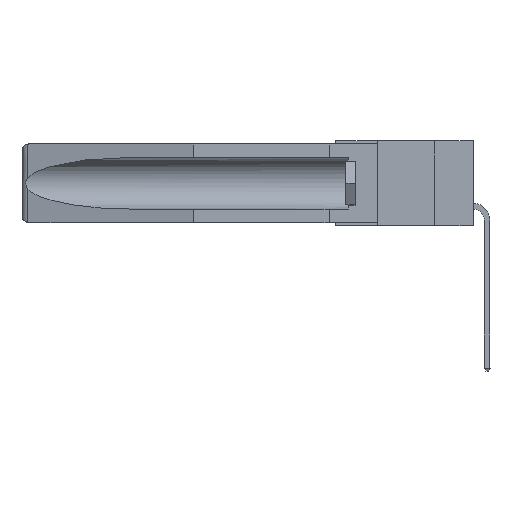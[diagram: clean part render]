
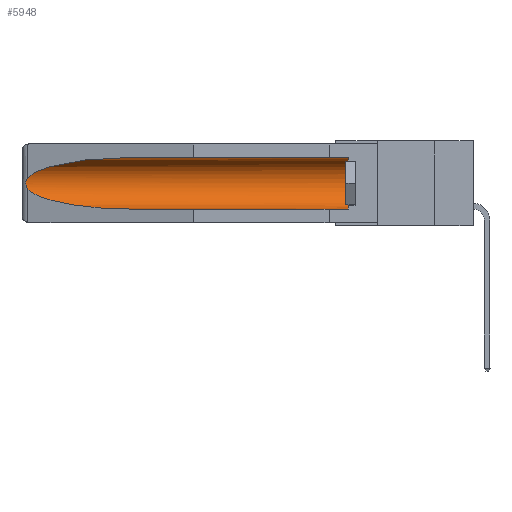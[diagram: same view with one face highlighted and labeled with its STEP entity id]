
A CAD part, left-side view. The second image highlights one B-rep face of the part: STEP entity #5948.
In plain terms, the highlighted cylindrical face has radius 2.857 mm (diameter 5.715 mm), a partial arc.
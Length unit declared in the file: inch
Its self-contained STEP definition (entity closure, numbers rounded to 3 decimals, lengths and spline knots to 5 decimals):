
#572 = CARTESIAN_POINT ( 'NONE',  ( 0.21114, 1.30732, -0.284 ) ) ;
#575 = ORIENTED_EDGE ( 'NONE', *, *, #4611, .T. ) ;
#780 = VERTEX_POINT ( 'NONE', #11968 ) ;
#1083 = EDGE_CURVE ( 'NONE', #9374, #9616, #26352, .T. ) ;
#1348 = CARTESIAN_POINT ( 'NONE',  ( 0.2675, 1.53308, -0.16763 ) ) ;
#1921 = CARTESIAN_POINT ( 'NONE',  ( 0.21114, 1.30732, -0.059 ) ) ;
#2210 = CARTESIAN_POINT ( 'NONE',  ( 0.155, 1.07973, -0.284 ) ) ;
#2550 = EDGE_LOOP ( 'NONE', ( #8007, #18191, #14293, #14109, #11131, #575 ) ) ;
#2733 = DIRECTION ( 'NONE',  ( 0., 0., 1. ) ) ;
#3683 = LINE ( 'NONE', #10826, #23333 ) ;
#4297 =( BOUNDED_CURVE ( )  B_SPLINE_CURVE ( 3, ( #20562, #16337, #572, #22596 ),
 .UNSPECIFIED., .F., .F. ) 
 B_SPLINE_CURVE_WITH_KNOTS ( ( 4, 4 ),
 ( 0.1948, 1.5708 ),
 .UNSPECIFIED. ) 
 CURVE ( )  GEOMETRIC_REPRESENTATION_ITEM ( )  RATIONAL_B_SPLINE_CURVE ( ( 1., 0.848, 0.848, 1. ) ) 
 REPRESENTATION_ITEM ( '' )  );
#4358 = CYLINDRICAL_SURFACE ( 'NONE', #18784, 0.1125 ) ;
#4552 = DIRECTION ( 'NONE',  ( 0., 0., 1. ) ) ;
#4611 = EDGE_CURVE ( 'NONE', #9616, #21609, #3683, .T. ) ;
#4628 = CARTESIAN_POINT ( 'NONE',  ( 0.155, 1.07973, -0.059 ) ) ;
#5948 = ADVANCED_FACE ( 'NONE', ( #7500 ), #4358, .F. ) ;
#7500 = FACE_OUTER_BOUND ( 'NONE', #2550, .T. ) ;
#8007 = ORIENTED_EDGE ( 'NONE', *, *, #20783, .T. ) ;
#8088 = CARTESIAN_POINT ( 'NONE',  ( 0.26597, 1.52961, -0.15275 ) ) ;
#8586 = CARTESIAN_POINT ( 'NONE',  ( 0.155, -0.30754, -0.284 ) ) ;
#8942 = AXIS2_PLACEMENT_3D ( 'NONE', #10487, #15095, #2733 ) ;
#9217 = CARTESIAN_POINT ( 'NONE',  ( 0.26537, 1.52718, -0.14972 ) ) ;
#9374 = VERTEX_POINT ( 'NONE', #22408 ) ;
#9489 = VECTOR ( 'NONE', #13034, 39.37008 ) ;
#9616 = VERTEX_POINT ( 'NONE', #27689 ) ;
#10418 = EDGE_CURVE ( 'NONE', #780, #18992, #4297, .T. ) ;
#10487 = CARTESIAN_POINT ( 'NONE',  ( 0.155, 0.126, -0.1715 ) ) ;
#10752 = EDGE_CURVE ( 'NONE', #9374, #18992, #13707, .T. ) ;
#10826 = CARTESIAN_POINT ( 'NONE',  ( 0.155, -0.30754, -0.059 ) ) ;
#11131 = ORIENTED_EDGE ( 'NONE', *, *, #1083, .T. ) ;
#11512 = EDGE_CURVE ( 'NONE', #20494, #780, #26389, .T. ) ;
#11968 = CARTESIAN_POINT ( 'NONE',  ( 0.26537, 1.52718, -0.19328 ) ) ;
#13034 = DIRECTION ( 'NONE',  ( 0., 1., 0. ) ) ;
#13707 = LINE ( 'NONE', #8586, #9489 ) ;
#14109 = ORIENTED_EDGE ( 'NONE', *, *, #10752, .F. ) ;
#14293 = ORIENTED_EDGE ( 'NONE', *, *, #10418, .T. ) ;
#15095 = DIRECTION ( 'NONE',  ( 0., -1., 0. ) ) ;
#15557 = CARTESIAN_POINT ( 'NONE',  ( 0.25451, 1.48313, -0.09465 ) ) ;
#16337 = CARTESIAN_POINT ( 'NONE',  ( 0.25451, 1.48313, -0.24835 ) ) ;
#16644 = CARTESIAN_POINT ( 'NONE',  ( 0.2673, 1.5327, -0.16383 ) ) ;
#17030 = CARTESIAN_POINT ( 'NONE',  ( 0.26597, 1.5296, -0.19026 ) ) ;
#17211 = DIRECTION ( 'NONE',  ( 0., 1., 0. ) ) ;
#17775 = CARTESIAN_POINT ( 'NONE',  ( 0.155, -0.30754, -0.1715 ) ) ;
#18191 = ORIENTED_EDGE ( 'NONE', *, *, #11512, .T. ) ;
#18784 = AXIS2_PLACEMENT_3D ( 'NONE', #17775, #24529, #4552 ) ;
#18874 = CARTESIAN_POINT ( 'NONE',  ( 0.26655, 1.53094, -0.18657 ) ) ;
#18992 = VERTEX_POINT ( 'NONE', #2210 ) ;
#19071 = CARTESIAN_POINT ( 'NONE',  ( 0.2675, 1.53308, -0.17534 ) ) ;
#20494 = VERTEX_POINT ( 'NONE', #9217 ) ;
#20562 = CARTESIAN_POINT ( 'NONE',  ( 0.26537, 1.52718, -0.19328 ) ) ;
#20783 = EDGE_CURVE ( 'NONE', #21609, #20494, #27646, .T. ) ;
#21609 = VERTEX_POINT ( 'NONE', #4628 ) ;
#22408 = CARTESIAN_POINT ( 'NONE',  ( 0.155, 0.126, -0.284 ) ) ;
#22596 = CARTESIAN_POINT ( 'NONE',  ( 0.155, 1.07973, -0.284 ) ) ;
#23333 = VECTOR ( 'NONE', #17211, 39.37008 ) ;
#24529 = DIRECTION ( 'NONE',  ( 0., 1., 0. ) ) ;
#24635 = CARTESIAN_POINT ( 'NONE',  ( 0.26537, 1.52718, -0.14972 ) ) ;
#25525 = CARTESIAN_POINT ( 'NONE',  ( 0.26537, 1.52718, -0.14972 ) ) ;
#25625 = CARTESIAN_POINT ( 'NONE',  ( 0.26537, 1.52718, -0.19328 ) ) ;
#25831 = CARTESIAN_POINT ( 'NONE',  ( 0.2673, 1.53269, -0.17917 ) ) ;
#26352 = CIRCLE ( 'NONE', #8942, 0.1125 ) ;
#26389 = B_SPLINE_CURVE_WITH_KNOTS ( 'NONE', 3,
 ( #25525, #8088, #27791, #16644, #1348, #19071, #25831, #18874, #17030, #25625 ),
 .UNSPECIFIED., .F., .F.,
 ( 4, 2, 2, 2, 4 ),
 ( 0., 0.00029, 0.00058, 0.00087, 0.00117 ),
 .UNSPECIFIED. ) ;
#26606 = CARTESIAN_POINT ( 'NONE',  ( 0.155, 1.07973, -0.059 ) ) ;
#27646 =( BOUNDED_CURVE ( )  B_SPLINE_CURVE ( 3, ( #26606, #1921, #15557, #24635 ),
 .UNSPECIFIED., .F., .F. ) 
 B_SPLINE_CURVE_WITH_KNOTS ( ( 4, 4 ),
 ( 4.71239, 6.08839 ),
 .UNSPECIFIED. ) 
 CURVE ( )  GEOMETRIC_REPRESENTATION_ITEM ( )  RATIONAL_B_SPLINE_CURVE ( ( 1., 0.848, 0.848, 1. ) ) 
 REPRESENTATION_ITEM ( '' )  );
#27689 = CARTESIAN_POINT ( 'NONE',  ( 0.155, 0.126, -0.059 ) ) ;
#27791 = CARTESIAN_POINT ( 'NONE',  ( 0.26654, 1.53092, -0.15636 ) ) ;
